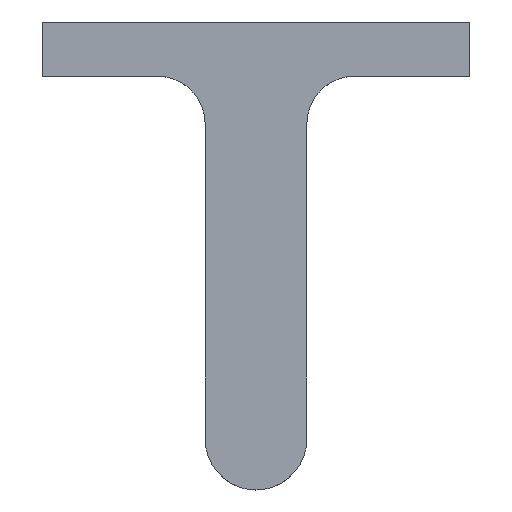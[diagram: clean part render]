
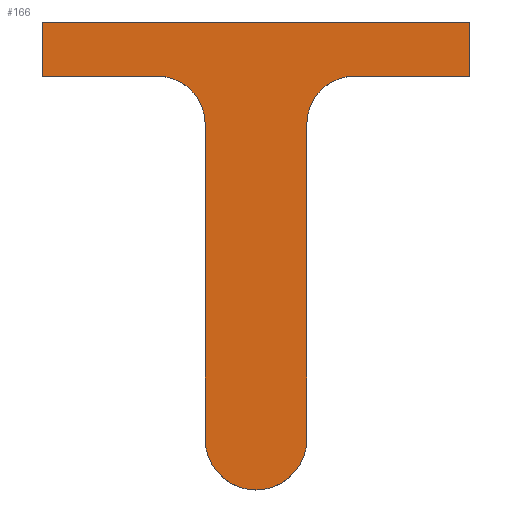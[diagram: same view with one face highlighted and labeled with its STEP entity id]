
A CAD part, top view. The second image highlights one B-rep face of the part: STEP entity #166.
In plain terms, the highlighted planar face has unit normal (0, 0, 1).
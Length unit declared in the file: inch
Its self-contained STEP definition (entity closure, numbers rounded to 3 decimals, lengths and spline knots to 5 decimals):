
#5 = DIRECTION ( 'NONE',  ( 1., 0., 0. ) ) ;
#6 = VERTEX_POINT ( 'NONE', #252 ) ;
#9 = ORIENTED_EDGE ( 'NONE', *, *, #75, .T. ) ;
#16 = CARTESIAN_POINT ( 'NONE',  ( 0., -0.3075, 0.015 ) ) ;
#17 = VECTOR ( 'NONE', #335, 39.37008 ) ;
#23 = CARTESIAN_POINT ( 'NONE',  ( 0.0375, -0.075, 0.015 ) ) ;
#25 = LINE ( 'NONE', #307, #190 ) ;
#35 = CARTESIAN_POINT ( 'NONE',  ( 0., -0.3075, 0.015 ) ) ;
#41 = CARTESIAN_POINT ( 'NONE',  ( -0.0725, -0.075, 0.015 ) ) ;
#43 = EDGE_CURVE ( 'NONE', #180, #295, #350, .T. ) ;
#55 = CARTESIAN_POINT ( 'NONE',  ( 0.1575, -0.04, 0.015 ) ) ;
#58 = EDGE_CURVE ( 'NONE', #295, #91, #310, .T. ) ;
#66 = LINE ( 'NONE', #365, #291 ) ;
#74 = ORIENTED_EDGE ( 'NONE', *, *, #264, .T. ) ;
#75 = EDGE_CURVE ( 'NONE', #355, #367, #154, .T. ) ;
#81 = ORIENTED_EDGE ( 'NONE', *, *, #58, .T. ) ;
#82 = DIRECTION ( 'NONE',  ( 1., 0., 0. ) ) ;
#83 = ORIENTED_EDGE ( 'NONE', *, *, #207, .T. ) ;
#88 = ORIENTED_EDGE ( 'NONE', *, *, #96, .T. ) ;
#89 = CARTESIAN_POINT ( 'NONE',  ( 0.0375, -0.075, 0.015 ) ) ;
#91 = VERTEX_POINT ( 'NONE', #159 ) ;
#93 = DIRECTION ( 'NONE',  ( 0., 1., 0. ) ) ;
#96 = EDGE_CURVE ( 'NONE', #367, #180, #25, .T. ) ;
#103 = CIRCLE ( 'NONE', #389, 0.035 ) ;
#105 = VECTOR ( 'NONE', #403, 39.37008 ) ;
#109 = CARTESIAN_POINT ( 'NONE',  ( 0.1575, -0.04, 0.015 ) ) ;
#111 = CARTESIAN_POINT ( 'NONE',  ( -0.0375, -0.3075, 0.015 ) ) ;
#113 = CARTESIAN_POINT ( 'NONE',  ( 0.1575, 0., 0.015 ) ) ;
#130 = AXIS2_PLACEMENT_3D ( 'NONE', #35, #192, #168 ) ;
#137 = DIRECTION ( 'NONE',  ( 0., -1., 0. ) ) ;
#146 = VERTEX_POINT ( 'NONE', #89 ) ;
#154 = LINE ( 'NONE', #280, #408 ) ;
#159 = CARTESIAN_POINT ( 'NONE',  ( -0.0725, -0.04, 0.015 ) ) ;
#166 = ADVANCED_FACE ( 'NONE', ( #203 ), #387, .T. ) ;
#168 = DIRECTION ( 'NONE',  ( 1., 0., 0. ) ) ;
#173 = DIRECTION ( 'NONE',  ( 0., 0., -1. ) ) ;
#180 = VERTEX_POINT ( 'NONE', #224 ) ;
#190 = VECTOR ( 'NONE', #380, 39.37008 ) ;
#192 = DIRECTION ( 'NONE',  ( 0., 0., 1. ) ) ;
#198 = VECTOR ( 'NONE', #5, 39.37008 ) ;
#203 = FACE_OUTER_BOUND ( 'NONE', #269, .T. ) ;
#207 = EDGE_CURVE ( 'NONE', #364, #355, #230, .T. ) ;
#209 = LINE ( 'NONE', #23, #105 ) ;
#213 = VERTEX_POINT ( 'NONE', #353 ) ;
#220 = EDGE_CURVE ( 'NONE', #213, #263, #66, .T. ) ;
#223 = AXIS2_PLACEMENT_3D ( 'NONE', #16, #393, #256 ) ;
#224 = CARTESIAN_POINT ( 'NONE',  ( -0.1575, 0., 0.015 ) ) ;
#230 = LINE ( 'NONE', #109, #198 ) ;
#232 = ORIENTED_EDGE ( 'NONE', *, *, #384, .T. ) ;
#233 = VECTOR ( 'NONE', #344, 39.37008 ) ;
#235 = EDGE_CURVE ( 'NONE', #263, #6, #333, .T. ) ;
#236 = CARTESIAN_POINT ( 'NONE',  ( -0.1575, -0.04, 0.015 ) ) ;
#243 = CARTESIAN_POINT ( 'NONE',  ( 0.0725, -0.075, 0.015 ) ) ;
#251 = CARTESIAN_POINT ( 'NONE',  ( -0.1575, -0.04, 0.015 ) ) ;
#252 = CARTESIAN_POINT ( 'NONE',  ( 0.0375, -0.3075, 0.015 ) ) ;
#256 = DIRECTION ( 'NONE',  ( 1., 0., 0. ) ) ;
#263 = VERTEX_POINT ( 'NONE', #111 ) ;
#264 = EDGE_CURVE ( 'NONE', #91, #213, #372, .T. ) ;
#269 = EDGE_LOOP ( 'NONE', ( #357, #232, #272, #83, #9, #88, #326, #81, #74, #304 ) ) ;
#272 = ORIENTED_EDGE ( 'NONE', *, *, #371, .T. ) ;
#280 = CARTESIAN_POINT ( 'NONE',  ( 0.1575, 0., 0.015 ) ) ;
#289 = DIRECTION ( 'NONE',  ( -1., 0., 0. ) ) ;
#291 = VECTOR ( 'NONE', #137, 39.37008 ) ;
#295 = VERTEX_POINT ( 'NONE', #236 ) ;
#304 = ORIENTED_EDGE ( 'NONE', *, *, #220, .T. ) ;
#307 = CARTESIAN_POINT ( 'NONE',  ( -0.1575, 0., 0.015 ) ) ;
#310 = LINE ( 'NONE', #251, #233 ) ;
#321 = AXIS2_PLACEMENT_3D ( 'NONE', #41, #173, #289 ) ;
#326 = ORIENTED_EDGE ( 'NONE', *, *, #43, .T. ) ;
#333 = CIRCLE ( 'NONE', #130, 0.0375 ) ;
#335 = DIRECTION ( 'NONE',  ( 0., -1., 0. ) ) ;
#336 = CARTESIAN_POINT ( 'NONE',  ( 0.0725, -0.04, 0.015 ) ) ;
#344 = DIRECTION ( 'NONE',  ( 1., 0., 0. ) ) ;
#350 = LINE ( 'NONE', #370, #17 ) ;
#353 = CARTESIAN_POINT ( 'NONE',  ( -0.0375, -0.075, 0.015 ) ) ;
#355 = VERTEX_POINT ( 'NONE', #55 ) ;
#357 = ORIENTED_EDGE ( 'NONE', *, *, #235, .T. ) ;
#364 = VERTEX_POINT ( 'NONE', #336 ) ;
#365 = CARTESIAN_POINT ( 'NONE',  ( -0.0375, -0.075, 0.015 ) ) ;
#367 = VERTEX_POINT ( 'NONE', #113 ) ;
#370 = CARTESIAN_POINT ( 'NONE',  ( -0.1575, 0., 0.015 ) ) ;
#371 = EDGE_CURVE ( 'NONE', #146, #364, #103, .T. ) ;
#372 = CIRCLE ( 'NONE', #321, 0.035 ) ;
#380 = DIRECTION ( 'NONE',  ( -1., 0., 0. ) ) ;
#384 = EDGE_CURVE ( 'NONE', #6, #146, #209, .T. ) ;
#387 = PLANE ( 'NONE',  #223 ) ;
#389 = AXIS2_PLACEMENT_3D ( 'NONE', #243, #400, #82 ) ;
#393 = DIRECTION ( 'NONE',  ( 0., 0., 1. ) ) ;
#400 = DIRECTION ( 'NONE',  ( 0., 0., -1. ) ) ;
#403 = DIRECTION ( 'NONE',  ( 0., 1., 0. ) ) ;
#408 = VECTOR ( 'NONE', #93, 39.37008 ) ;
